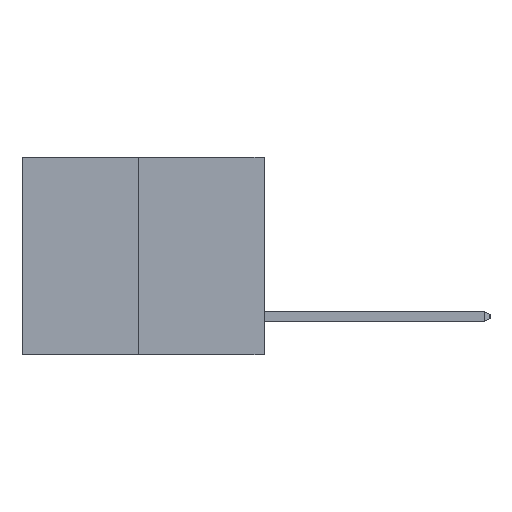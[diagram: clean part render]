
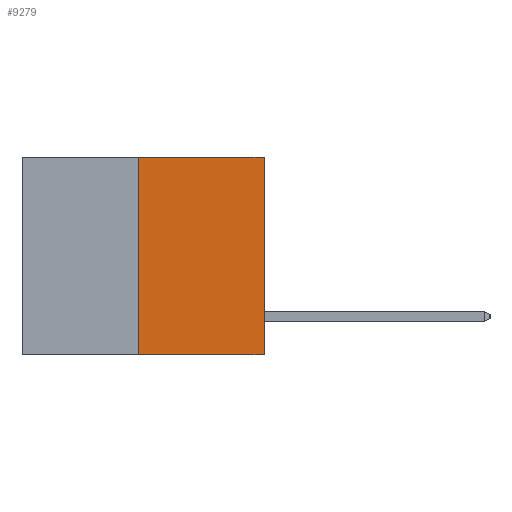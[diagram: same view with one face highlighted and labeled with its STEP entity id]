
A CAD part, left-side view. The second image highlights one B-rep face of the part: STEP entity #9279.
In plain terms, the highlighted planar face has unit normal (-1, 0, 0).
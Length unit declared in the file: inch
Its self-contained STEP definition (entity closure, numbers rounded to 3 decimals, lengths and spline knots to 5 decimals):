
#91 = PLANE ( 'NONE',  #4344 ) ;
#171 = DIRECTION ( 'NONE',  ( 0., 0., -1. ) ) ;
#1748 = VECTOR ( 'NONE', #5409, 39.37008 ) ;
#1769 = VERTEX_POINT ( 'NONE', #20885 ) ;
#1985 = LINE ( 'NONE', #16337, #8074 ) ;
#2258 = DIRECTION ( 'NONE',  ( 0., 0., 1. ) ) ;
#2461 = VECTOR ( 'NONE', #10763, 39.37008 ) ;
#2754 = VERTEX_POINT ( 'NONE', #16666 ) ;
#3173 = ORIENTED_EDGE ( 'NONE', *, *, #8254, .F. ) ;
#4034 = EDGE_LOOP ( 'NONE', ( #10351, #9178, #12089, #3173 ) ) ;
#4344 = AXIS2_PLACEMENT_3D ( 'NONE', #12503, #5428, #171 ) ;
#4512 = VERTEX_POINT ( 'NONE', #8409 ) ;
#5409 = DIRECTION ( 'NONE',  ( 0., 0., 1. ) ) ;
#5428 = DIRECTION ( 'NONE',  ( 1., 0., 0. ) ) ;
#7158 = LINE ( 'NONE', #19973, #2461 ) ;
#7690 = EDGE_CURVE ( 'NONE', #4512, #1769, #21212, .T. ) ;
#8074 = VECTOR ( 'NONE', #16255, 39.37008 ) ;
#8254 = EDGE_CURVE ( 'NONE', #12807, #1769, #1985, .T. ) ;
#8409 = CARTESIAN_POINT ( 'NONE',  ( 0., 0., -0.49 ) ) ;
#9178 = ORIENTED_EDGE ( 'NONE', *, *, #22174, .T. ) ;
#9279 = ADVANCED_FACE ( 'NONE', ( #14108 ), #91, .F. ) ;
#10351 = ORIENTED_EDGE ( 'NONE', *, *, #20092, .F. ) ;
#10759 = CARTESIAN_POINT ( 'NONE',  ( 0., 0.312, -0.49 ) ) ;
#10763 = DIRECTION ( 'NONE',  ( 0., -1., 0. ) ) ;
#11083 = CARTESIAN_POINT ( 'NONE',  ( 0., 0., 0. ) ) ;
#12089 = ORIENTED_EDGE ( 'NONE', *, *, #7690, .T. ) ;
#12503 = CARTESIAN_POINT ( 'NONE',  ( 0., 0.6, 0. ) ) ;
#12807 = VERTEX_POINT ( 'NONE', #13895 ) ;
#13895 = CARTESIAN_POINT ( 'NONE',  ( 0., 0.312, 0. ) ) ;
#14108 = FACE_OUTER_BOUND ( 'NONE', #4034, .T. ) ;
#16255 = DIRECTION ( 'NONE',  ( 0., -1., 0. ) ) ;
#16337 = CARTESIAN_POINT ( 'NONE',  ( 0., 0.6, 0. ) ) ;
#16666 = CARTESIAN_POINT ( 'NONE',  ( 0., 0.312, -0.49 ) ) ;
#19973 = CARTESIAN_POINT ( 'NONE',  ( 0., 0.6, -0.49 ) ) ;
#20092 = EDGE_CURVE ( 'NONE', #2754, #12807, #20111, .T. ) ;
#20111 = LINE ( 'NONE', #10759, #1748 ) ;
#20885 = CARTESIAN_POINT ( 'NONE',  ( 0., 0., 0. ) ) ;
#21212 = LINE ( 'NONE', #11083, #22336 ) ;
#22174 = EDGE_CURVE ( 'NONE', #2754, #4512, #7158, .T. ) ;
#22336 = VECTOR ( 'NONE', #2258, 39.37008 ) ;
